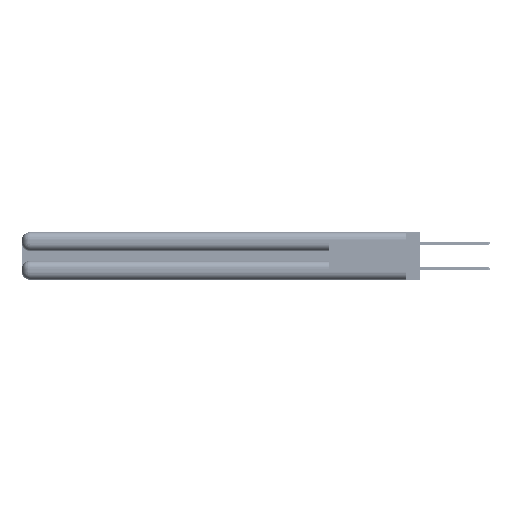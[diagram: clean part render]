
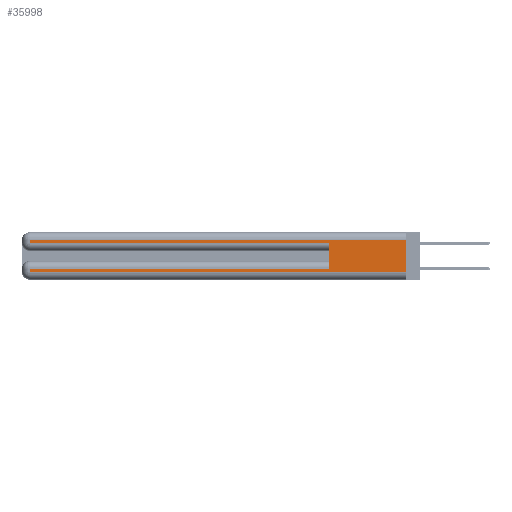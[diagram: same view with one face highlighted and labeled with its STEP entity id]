
A CAD part, left-side view. The second image highlights one B-rep face of the part: STEP entity #35998.
In plain terms, the highlighted planar face has unit normal (-1, 0, 0).
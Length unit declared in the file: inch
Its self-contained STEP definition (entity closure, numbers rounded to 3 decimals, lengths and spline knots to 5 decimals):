
#126 = CARTESIAN_POINT ( 'NONE',  ( 0., 0., 0.06 ) ) ;
#1217 = VECTOR ( 'NONE', #47370, 39.37008 ) ;
#3346 = DIRECTION ( 'NONE',  ( 0., 1., 0. ) ) ;
#5373 = CARTESIAN_POINT ( 'NONE',  ( 0., 0.6, 0.285 ) ) ;
#5857 = CARTESIAN_POINT ( 'NONE',  ( 0., 2.94, 0.285 ) ) ;
#6528 = PLANE ( 'NONE',  #9567 ) ;
#6916 = CARTESIAN_POINT ( 'NONE',  ( 0., 0.6, 0.085 ) ) ;
#7581 = EDGE_CURVE ( 'NONE', #54423, #18305, #52899, .T. ) ;
#7895 = CARTESIAN_POINT ( 'NONE',  ( 0., 2.94, 0.37 ) ) ;
#9263 = VERTEX_POINT ( 'NONE', #126 ) ;
#9433 = ORIENTED_EDGE ( 'NONE', *, *, #12951, .F. ) ;
#9567 = AXIS2_PLACEMENT_3D ( 'NONE', #53275, #36554, #10900 ) ;
#10177 = CARTESIAN_POINT ( 'NONE',  ( 0., 0., 0.285 ) ) ;
#10667 = ORIENTED_EDGE ( 'NONE', *, *, #44840, .T. ) ;
#10900 = DIRECTION ( 'NONE',  ( 0., 0., -1. ) ) ;
#10927 = ORIENTED_EDGE ( 'NONE', *, *, #32239, .T. ) ;
#11224 = ORIENTED_EDGE ( 'NONE', *, *, #13720, .T. ) ;
#12685 = LINE ( 'NONE', #10177, #22782 ) ;
#12951 = EDGE_CURVE ( 'NONE', #44972, #9263, #51342, .T. ) ;
#13720 = EDGE_CURVE ( 'NONE', #33809, #18305, #12685, .T. ) ;
#13935 = DIRECTION ( 'NONE',  ( 0., 0., 1. ) ) ;
#14167 = ORIENTED_EDGE ( 'NONE', *, *, #7581, .F. ) ;
#14215 = ORIENTED_EDGE ( 'NONE', *, *, #20753, .T. ) ;
#14315 = ORIENTED_EDGE ( 'NONE', *, *, #42214, .T. ) ;
#16110 = ORIENTED_EDGE ( 'NONE', *, *, #41668, .T. ) ;
#16918 = CARTESIAN_POINT ( 'NONE',  ( 0., 2.94, 0.085 ) ) ;
#17946 = DIRECTION ( 'NONE',  ( 0., 0., -1. ) ) ;
#18305 = VERTEX_POINT ( 'NONE', #5373 ) ;
#20425 = VERTEX_POINT ( 'NONE', #31422 ) ;
#20753 = EDGE_CURVE ( 'NONE', #54423, #23984, #54608, .T. ) ;
#21995 = CARTESIAN_POINT ( 'NONE',  ( 0., 0., 0.31 ) ) ;
#22003 = CARTESIAN_POINT ( 'NONE',  ( 0., 2.94, 0.37 ) ) ;
#22204 = VECTOR ( 'NONE', #3346, 39.37008 ) ;
#22730 = CARTESIAN_POINT ( 'NONE',  ( 0., 0., 0.31 ) ) ;
#22782 = VECTOR ( 'NONE', #44303, 39.37008 ) ;
#23984 = VERTEX_POINT ( 'NONE', #16918 ) ;
#24360 = VECTOR ( 'NONE', #29370, 39.37008 ) ;
#24990 = VECTOR ( 'NONE', #17946, 39.37008 ) ;
#25578 = LINE ( 'NONE', #27304, #46719 ) ;
#26325 = DIRECTION ( 'NONE',  ( 0., 1., 0. ) ) ;
#26899 = CARTESIAN_POINT ( 'NONE',  ( 0., 0.6, 0.145 ) ) ;
#27068 = LINE ( 'NONE', #7895, #24360 ) ;
#27304 = CARTESIAN_POINT ( 'NONE',  ( 0., 0., 0.06 ) ) ;
#29155 = CARTESIAN_POINT ( 'NONE',  ( 0., 0., 0.085 ) ) ;
#29370 = DIRECTION ( 'NONE',  ( 0., 0., -1. ) ) ;
#29865 = CARTESIAN_POINT ( 'NONE',  ( 0., 2.94, 0.31 ) ) ;
#31422 = CARTESIAN_POINT ( 'NONE',  ( 0., 2.94, 0.06 ) ) ;
#31592 = DIRECTION ( 'NONE',  ( 0., -1., 0. ) ) ;
#32239 = EDGE_CURVE ( 'NONE', #38607, #33809, #27068, .T. ) ;
#33809 = VERTEX_POINT ( 'NONE', #5857 ) ;
#35174 = VECTOR ( 'NONE', #26325, 39.37008 ) ;
#35998 = ADVANCED_FACE ( 'NONE', ( #37610 ), #6528, .F. ) ;
#36554 = DIRECTION ( 'NONE',  ( 1., 0., 0. ) ) ;
#37610 = FACE_OUTER_BOUND ( 'NONE', #49362, .T. ) ;
#38607 = VERTEX_POINT ( 'NONE', #29865 ) ;
#41668 = EDGE_CURVE ( 'NONE', #20425, #9263, #25578, .T. ) ;
#42214 = EDGE_CURVE ( 'NONE', #23984, #20425, #42708, .T. ) ;
#42708 = LINE ( 'NONE', #22003, #1217 ) ;
#43549 = CARTESIAN_POINT ( 'NONE',  ( 0., 0., 0.37 ) ) ;
#44303 = DIRECTION ( 'NONE',  ( 0., -1., 0. ) ) ;
#44840 = EDGE_CURVE ( 'NONE', #44972, #38607, #46369, .T. ) ;
#44972 = VERTEX_POINT ( 'NONE', #22730 ) ;
#46369 = LINE ( 'NONE', #21995, #35174 ) ;
#46719 = VECTOR ( 'NONE', #31592, 39.37008 ) ;
#47370 = DIRECTION ( 'NONE',  ( 0., 0., -1. ) ) ;
#49362 = EDGE_LOOP ( 'NONE', ( #9433, #10667, #10927, #11224, #14167, #14215, #14315, #16110 ) ) ;
#51342 = LINE ( 'NONE', #43549, #24990 ) ;
#51573 = VECTOR ( 'NONE', #13935, 39.37008 ) ;
#52899 = LINE ( 'NONE', #26899, #51573 ) ;
#53275 = CARTESIAN_POINT ( 'NONE',  ( 0., 0., 0.37 ) ) ;
#54423 = VERTEX_POINT ( 'NONE', #6916 ) ;
#54608 = LINE ( 'NONE', #29155, #22204 ) ;
